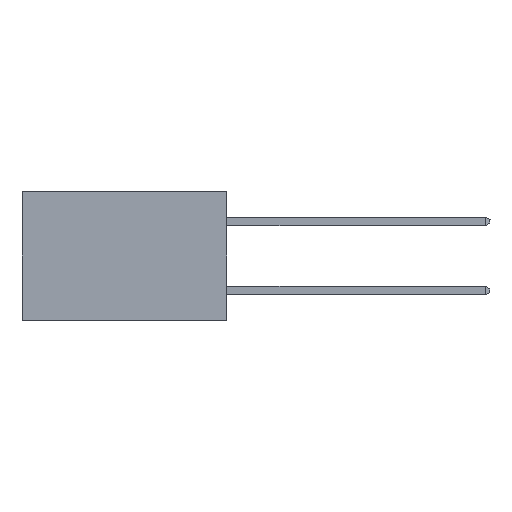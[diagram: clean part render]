
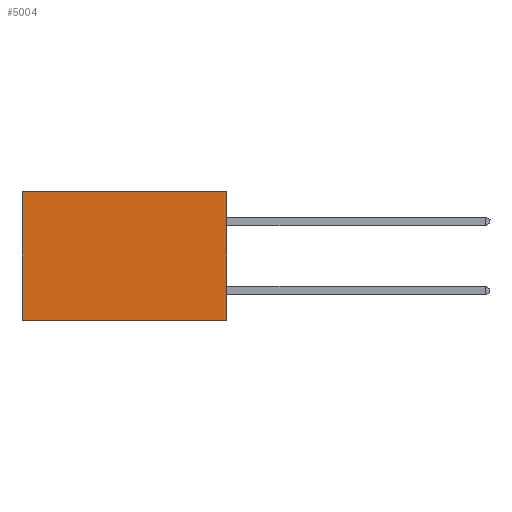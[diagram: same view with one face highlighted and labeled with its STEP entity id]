
A CAD part, left-side view. The second image highlights one B-rep face of the part: STEP entity #5004.
In plain terms, the highlighted planar face has unit normal (-1, 0, 0).
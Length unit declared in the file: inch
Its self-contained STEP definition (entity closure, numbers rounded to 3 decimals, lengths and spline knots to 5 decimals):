
#290 = DIRECTION ( 'NONE',  ( 0., 0., -1. ) ) ;
#680 = VECTOR ( 'NONE', #5539, 39.37008 ) ;
#1319 = VECTOR ( 'NONE', #5044, 39.37008 ) ;
#1698 = EDGE_CURVE ( 'NONE', #6494, #1838, #2958, .T. ) ;
#1782 = EDGE_LOOP ( 'NONE', ( #4324, #4545, #4720, #4731 ) ) ;
#1838 = VERTEX_POINT ( 'NONE', #7206 ) ;
#1882 = AXIS2_PLACEMENT_3D ( 'NONE', #4507, #2926, #8350 ) ;
#2802 = LINE ( 'NONE', #8435, #680 ) ;
#2926 = DIRECTION ( 'NONE',  ( 1., 0., 0. ) ) ;
#2958 = LINE ( 'NONE', #5962, #6882 ) ;
#3706 = LINE ( 'NONE', #5844, #1319 ) ;
#3789 = VERTEX_POINT ( 'NONE', #6821 ) ;
#4284 = CARTESIAN_POINT ( 'NONE',  ( 0.277, 0., 0. ) ) ;
#4324 = ORIENTED_EDGE ( 'NONE', *, *, #5853, .T. ) ;
#4507 = CARTESIAN_POINT ( 'NONE',  ( 0.277, 0., -0.37 ) ) ;
#4545 = ORIENTED_EDGE ( 'NONE', *, *, #1698, .F. ) ;
#4720 = ORIENTED_EDGE ( 'NONE', *, *, #9353, .F. ) ;
#4731 = ORIENTED_EDGE ( 'NONE', *, *, #8021, .T. ) ;
#4878 = DIRECTION ( 'NONE',  ( 0., 1., 0. ) ) ;
#5004 = ADVANCED_FACE ( 'NONE', ( #6070 ), #9795, .F. ) ;
#5044 = DIRECTION ( 'NONE',  ( 0., 1., 0. ) ) ;
#5090 = LINE ( 'NONE', #8843, #6838 ) ;
#5539 = DIRECTION ( 'NONE',  ( 0., 0., -1. ) ) ;
#5844 = CARTESIAN_POINT ( 'NONE',  ( 0.277, 0., 0. ) ) ;
#5853 = EDGE_CURVE ( 'NONE', #3789, #1838, #5090, .T. ) ;
#5962 = CARTESIAN_POINT ( 'NONE',  ( 0.277, 0., -0.37 ) ) ;
#6070 = FACE_OUTER_BOUND ( 'NONE', #1782, .T. ) ;
#6360 = CARTESIAN_POINT ( 'NONE',  ( 0.277, 0., -0.37 ) ) ;
#6494 = VERTEX_POINT ( 'NONE', #6360 ) ;
#6792 = VERTEX_POINT ( 'NONE', #4284 ) ;
#6821 = CARTESIAN_POINT ( 'NONE',  ( 0.277, 0.59, 0. ) ) ;
#6838 = VECTOR ( 'NONE', #290, 39.37008 ) ;
#6882 = VECTOR ( 'NONE', #4878, 39.37008 ) ;
#7206 = CARTESIAN_POINT ( 'NONE',  ( 0.277, 0.59, -0.37 ) ) ;
#8021 = EDGE_CURVE ( 'NONE', #6792, #3789, #3706, .T. ) ;
#8350 = DIRECTION ( 'NONE',  ( 0., 0., -1. ) ) ;
#8435 = CARTESIAN_POINT ( 'NONE',  ( 0.277, 0., -0.37 ) ) ;
#8843 = CARTESIAN_POINT ( 'NONE',  ( 0.277, 0.59, -0.37 ) ) ;
#9353 = EDGE_CURVE ( 'NONE', #6792, #6494, #2802, .T. ) ;
#9795 = PLANE ( 'NONE',  #1882 ) ;
